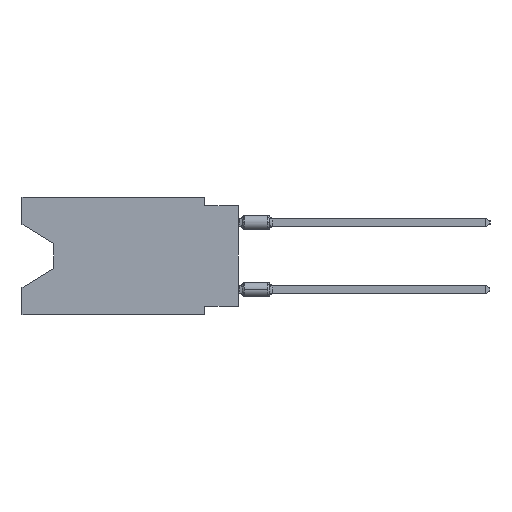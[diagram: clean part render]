
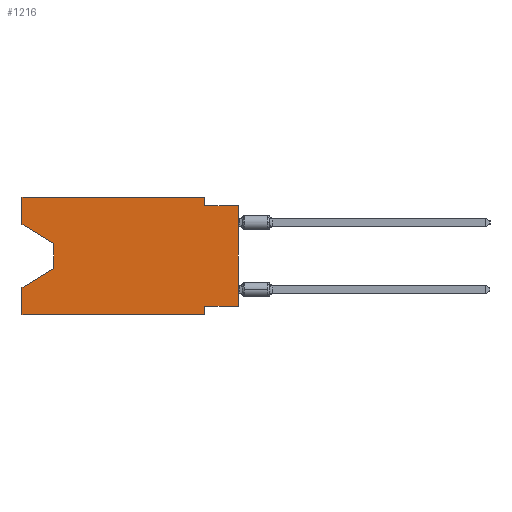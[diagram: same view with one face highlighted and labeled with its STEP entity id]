
A CAD part, left-side view. The second image highlights one B-rep face of the part: STEP entity #1216.
In plain terms, the highlighted planar face has unit normal (-1, 0, 0).
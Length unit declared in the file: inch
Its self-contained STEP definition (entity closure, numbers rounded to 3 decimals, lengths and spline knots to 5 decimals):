
#105 = VERTEX_POINT ( 'NONE', #58472 ) ;
#579 = ORIENTED_EDGE ( 'NONE', *, *, #24696, .T. ) ;
#1144 = VECTOR ( 'NONE', #48215, 39.37008 ) ;
#1216 = ADVANCED_FACE ( 'NONE', ( #16792 ), #58173, .F. ) ;
#1749 = EDGE_CURVE ( 'NONE', #15658, #6864, #35072, .T. ) ;
#1886 = VERTEX_POINT ( 'NONE', #60512 ) ;
#2774 = CARTESIAN_POINT ( 'NONE',  ( 0., 0.645, 0. ) ) ;
#4380 = DIRECTION ( 'NONE',  ( 0., -0.855, -0.519 ) ) ;
#4994 = EDGE_CURVE ( 'NONE', #1886, #15658, #27735, .T. ) ;
#5147 = VECTOR ( 'NONE', #10384, 39.37008 ) ;
#5194 = LINE ( 'NONE', #47197, #44150 ) ;
#5861 = DIRECTION ( 'NONE',  ( 0., -1., 0. ) ) ;
#6864 = VERTEX_POINT ( 'NONE', #33851 ) ;
#6983 = CARTESIAN_POINT ( 'NONE',  ( 0., 0.1, -0.025 ) ) ;
#7690 = EDGE_CURVE ( 'NONE', #31114, #15052, #13845, .T. ) ;
#8411 = AXIS2_PLACEMENT_3D ( 'NONE', #2774, #53497, #54402 ) ;
#8546 = ORIENTED_EDGE ( 'NONE', *, *, #1749, .F. ) ;
#9069 = ORIENTED_EDGE ( 'NONE', *, *, #4994, .F. ) ;
#9148 = EDGE_CURVE ( 'NONE', #15052, #28820, #25146, .T. ) ;
#10251 = CARTESIAN_POINT ( 'NONE',  ( 0., 0., -0.025 ) ) ;
#10384 = DIRECTION ( 'NONE',  ( 0., 0., -1. ) ) ;
#10411 = VECTOR ( 'NONE', #5861, 39.37008 ) ;
#13845 = LINE ( 'NONE', #38117, #35287 ) ;
#13922 = CARTESIAN_POINT ( 'NONE',  ( 0., 0.645, -0.35 ) ) ;
#14210 = ORIENTED_EDGE ( 'NONE', *, *, #40073, .T. ) ;
#14727 = CARTESIAN_POINT ( 'NONE',  ( 0., 0.645, -0.35 ) ) ;
#14807 = CARTESIAN_POINT ( 'NONE',  ( 0., 0., 0. ) ) ;
#15043 = LINE ( 'NONE', #33101, #5147 ) ;
#15052 = VERTEX_POINT ( 'NONE', #23717 ) ;
#15658 = VERTEX_POINT ( 'NONE', #31292 ) ;
#16599 = ORIENTED_EDGE ( 'NONE', *, *, #9148, .F. ) ;
#16792 = FACE_OUTER_BOUND ( 'NONE', #19507, .T. ) ;
#17079 = VERTEX_POINT ( 'NONE', #6983 ) ;
#19507 = EDGE_LOOP ( 'NONE', ( #30816, #49172, #579, #51701, #57978, #8546, #9069, #14210, #33297, #27528, #16599, #60187 ) ) ;
#19676 = VECTOR ( 'NONE', #37886, 39.37008 ) ;
#22220 = CARTESIAN_POINT ( 'NONE',  ( 0., 0.645, -0.08025 ) ) ;
#22475 = EDGE_CURVE ( 'NONE', #53365, #6864, #47537, .T. ) ;
#23717 = CARTESIAN_POINT ( 'NONE',  ( 0., 0.645, 0. ) ) ;
#24342 = VECTOR ( 'NONE', #53406, 39.37008 ) ;
#24696 = EDGE_CURVE ( 'NONE', #31734, #105, #24961, .T. ) ;
#24961 = LINE ( 'NONE', #34281, #38789 ) ;
#25146 = LINE ( 'NONE', #29816, #10411 ) ;
#26226 = EDGE_CURVE ( 'NONE', #17079, #61099, #33900, .T. ) ;
#27123 = EDGE_CURVE ( 'NONE', #28820, #17079, #15043, .T. ) ;
#27528 = ORIENTED_EDGE ( 'NONE', *, *, #27123, .F. ) ;
#27735 = LINE ( 'NONE', #57761, #24342 ) ;
#28820 = VERTEX_POINT ( 'NONE', #61397 ) ;
#29816 = CARTESIAN_POINT ( 'NONE',  ( 0., 0.645, 0. ) ) ;
#30164 = VECTOR ( 'NONE', #34411, 39.37008 ) ;
#30816 = ORIENTED_EDGE ( 'NONE', *, *, #39537, .T. ) ;
#31114 = VERTEX_POINT ( 'NONE', #22220 ) ;
#31292 = CARTESIAN_POINT ( 'NONE',  ( 0., 0.1, -0.325 ) ) ;
#31734 = VERTEX_POINT ( 'NONE', #51666 ) ;
#33101 = CARTESIAN_POINT ( 'NONE',  ( 0., 0.1, 0. ) ) ;
#33297 = ORIENTED_EDGE ( 'NONE', *, *, #26226, .F. ) ;
#33851 = CARTESIAN_POINT ( 'NONE',  ( 0., 0.1, -0.35 ) ) ;
#33900 = LINE ( 'NONE', #10251, #1144 ) ;
#34281 = CARTESIAN_POINT ( 'NONE',  ( 0., 0.55, -0.212 ) ) ;
#34411 = DIRECTION ( 'NONE',  ( 0., 0., 1. ) ) ;
#34721 = VERTEX_POINT ( 'NONE', #41933 ) ;
#35072 = LINE ( 'NONE', #44426, #39943 ) ;
#35287 = VECTOR ( 'NONE', #56151, 39.37008 ) ;
#35721 = EDGE_CURVE ( 'NONE', #34721, #31734, #47704, .T. ) ;
#37886 = DIRECTION ( 'NONE',  ( 0., -1., 0. ) ) ;
#38117 = CARTESIAN_POINT ( 'NONE',  ( 0., 0.645, 0. ) ) ;
#38467 = LINE ( 'NONE', #14807, #30164 ) ;
#38789 = VECTOR ( 'NONE', #43300, 39.37008 ) ;
#39537 = EDGE_CURVE ( 'NONE', #31114, #34721, #59741, .T. ) ;
#39943 = VECTOR ( 'NONE', #54030, 39.37008 ) ;
#40073 = EDGE_CURVE ( 'NONE', #1886, #61099, #38467, .T. ) ;
#41933 = CARTESIAN_POINT ( 'NONE',  ( 0., 0.55, -0.138 ) ) ;
#42670 = VECTOR ( 'NONE', #43340, 39.37008 ) ;
#43130 = DIRECTION ( 'NONE',  ( 0., 0., 1. ) ) ;
#43300 = DIRECTION ( 'NONE',  ( 0., 0.855, -0.519 ) ) ;
#43340 = DIRECTION ( 'NONE',  ( 0., 0., -1. ) ) ;
#44150 = VECTOR ( 'NONE', #43130, 39.37008 ) ;
#44426 = CARTESIAN_POINT ( 'NONE',  ( 0., 0.1, -0.35 ) ) ;
#47053 = CARTESIAN_POINT ( 'NONE',  ( 0., 0., -0.025 ) ) ;
#47197 = CARTESIAN_POINT ( 'NONE',  ( 0., 0.645, 0. ) ) ;
#47537 = LINE ( 'NONE', #13922, #19676 ) ;
#47704 = LINE ( 'NONE', #57318, #42670 ) ;
#47783 = EDGE_CURVE ( 'NONE', #53365, #105, #5194, .T. ) ;
#48215 = DIRECTION ( 'NONE',  ( 0., -1., 0. ) ) ;
#49172 = ORIENTED_EDGE ( 'NONE', *, *, #35721, .T. ) ;
#50431 = CARTESIAN_POINT ( 'NONE',  ( 0., 0.645, -0.08025 ) ) ;
#51666 = CARTESIAN_POINT ( 'NONE',  ( 0., 0.55, -0.212 ) ) ;
#51701 = ORIENTED_EDGE ( 'NONE', *, *, #47783, .F. ) ;
#53365 = VERTEX_POINT ( 'NONE', #14727 ) ;
#53406 = DIRECTION ( 'NONE',  ( 0., 1., 0. ) ) ;
#53497 = DIRECTION ( 'NONE',  ( 1., 0., 0. ) ) ;
#54030 = DIRECTION ( 'NONE',  ( 0., 0., -1. ) ) ;
#54402 = DIRECTION ( 'NONE',  ( 0., 0., -1. ) ) ;
#56151 = DIRECTION ( 'NONE',  ( 0., 0., 1. ) ) ;
#56890 = VECTOR ( 'NONE', #4380, 39.37008 ) ;
#57318 = CARTESIAN_POINT ( 'NONE',  ( 0., 0.55, -0.138 ) ) ;
#57761 = CARTESIAN_POINT ( 'NONE',  ( 0., 0., -0.325 ) ) ;
#57978 = ORIENTED_EDGE ( 'NONE', *, *, #22475, .T. ) ;
#58173 = PLANE ( 'NONE',  #8411 ) ;
#58472 = CARTESIAN_POINT ( 'NONE',  ( 0., 0.645, -0.26975 ) ) ;
#59741 = LINE ( 'NONE', #50431, #56890 ) ;
#60187 = ORIENTED_EDGE ( 'NONE', *, *, #7690, .F. ) ;
#60512 = CARTESIAN_POINT ( 'NONE',  ( 0., 0., -0.325 ) ) ;
#61099 = VERTEX_POINT ( 'NONE', #47053 ) ;
#61397 = CARTESIAN_POINT ( 'NONE',  ( 0., 0.1, 0. ) ) ;
